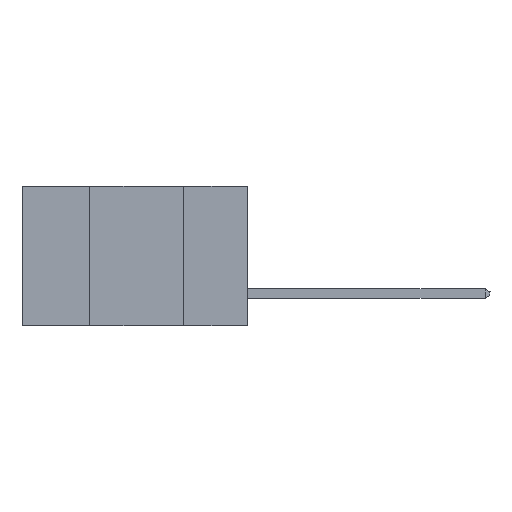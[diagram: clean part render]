
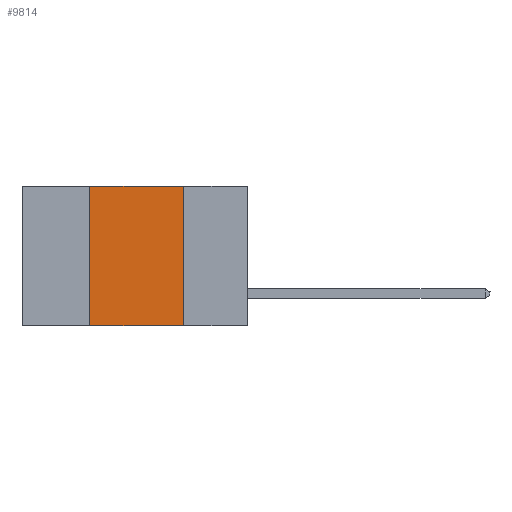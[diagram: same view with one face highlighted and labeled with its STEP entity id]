
A CAD part, left-side view. The second image highlights one B-rep face of the part: STEP entity #9814.
In plain terms, the highlighted planar face has unit normal (-1, 0, 0).
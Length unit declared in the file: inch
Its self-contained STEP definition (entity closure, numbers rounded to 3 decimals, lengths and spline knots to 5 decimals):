
#25 = CARTESIAN_POINT ( 'NONE',  ( 0., 0.17, -0.37 ) ) ;
#1010 = VECTOR ( 'NONE', #3035, 39.37008 ) ;
#1473 = AXIS2_PLACEMENT_3D ( 'NONE', #6976, #11445, #8583 ) ;
#1501 = DIRECTION ( 'NONE',  ( 0., -1., 0. ) ) ;
#1674 = ORIENTED_EDGE ( 'NONE', *, *, #9377, .T. ) ;
#2292 = VERTEX_POINT ( 'NONE', #25 ) ;
#2372 = EDGE_LOOP ( 'NONE', ( #10157, #16719, #12732, #1674 ) ) ;
#2836 = LINE ( 'NONE', #16333, #12341 ) ;
#3035 = DIRECTION ( 'NONE',  ( 0., 0., 1. ) ) ;
#4825 = CARTESIAN_POINT ( 'NONE',  ( 0., 0.17, -0.37 ) ) ;
#5757 = EDGE_CURVE ( 'NONE', #6988, #2292, #17327, .T. ) ;
#6976 = CARTESIAN_POINT ( 'NONE',  ( 0., 0.6, 0. ) ) ;
#6988 = VERTEX_POINT ( 'NONE', #7778 ) ;
#7337 = FACE_OUTER_BOUND ( 'NONE', #2372, .T. ) ;
#7778 = CARTESIAN_POINT ( 'NONE',  ( 0., 0.17, 0. ) ) ;
#8583 = DIRECTION ( 'NONE',  ( 0., 0., -1. ) ) ;
#8653 = CARTESIAN_POINT ( 'NONE',  ( 0., 0.42, -0.37 ) ) ;
#9377 = EDGE_CURVE ( 'NONE', #10340, #2292, #2836, .T. ) ;
#9409 = VECTOR ( 'NONE', #15814, 39.37008 ) ;
#9718 = EDGE_CURVE ( 'NONE', #13522, #6988, #11360, .T. ) ;
#9814 = ADVANCED_FACE ( 'NONE', ( #7337 ), #12793, .F. ) ;
#9836 = CARTESIAN_POINT ( 'NONE',  ( 0., 0.6, 0. ) ) ;
#10014 = LINE ( 'NONE', #15465, #1010 ) ;
#10157 = ORIENTED_EDGE ( 'NONE', *, *, #5757, .F. ) ;
#10340 = VERTEX_POINT ( 'NONE', #8653 ) ;
#11360 = LINE ( 'NONE', #9836, #14592 ) ;
#11445 = DIRECTION ( 'NONE',  ( 1., 0., 0. ) ) ;
#12341 = VECTOR ( 'NONE', #1501, 39.37008 ) ;
#12732 = ORIENTED_EDGE ( 'NONE', *, *, #15006, .F. ) ;
#12793 = PLANE ( 'NONE',  #1473 ) ;
#13522 = VERTEX_POINT ( 'NONE', #14495 ) ;
#13942 = DIRECTION ( 'NONE',  ( 0., -1., 0. ) ) ;
#14495 = CARTESIAN_POINT ( 'NONE',  ( 0., 0.42, 0. ) ) ;
#14592 = VECTOR ( 'NONE', #13942, 39.37008 ) ;
#15006 = EDGE_CURVE ( 'NONE', #10340, #13522, #10014, .T. ) ;
#15465 = CARTESIAN_POINT ( 'NONE',  ( 0., 0.42, -0.37 ) ) ;
#15814 = DIRECTION ( 'NONE',  ( 0., 0., -1. ) ) ;
#16333 = CARTESIAN_POINT ( 'NONE',  ( 0., 0.6, -0.37 ) ) ;
#16719 = ORIENTED_EDGE ( 'NONE', *, *, #9718, .F. ) ;
#17327 = LINE ( 'NONE', #4825, #9409 ) ;
